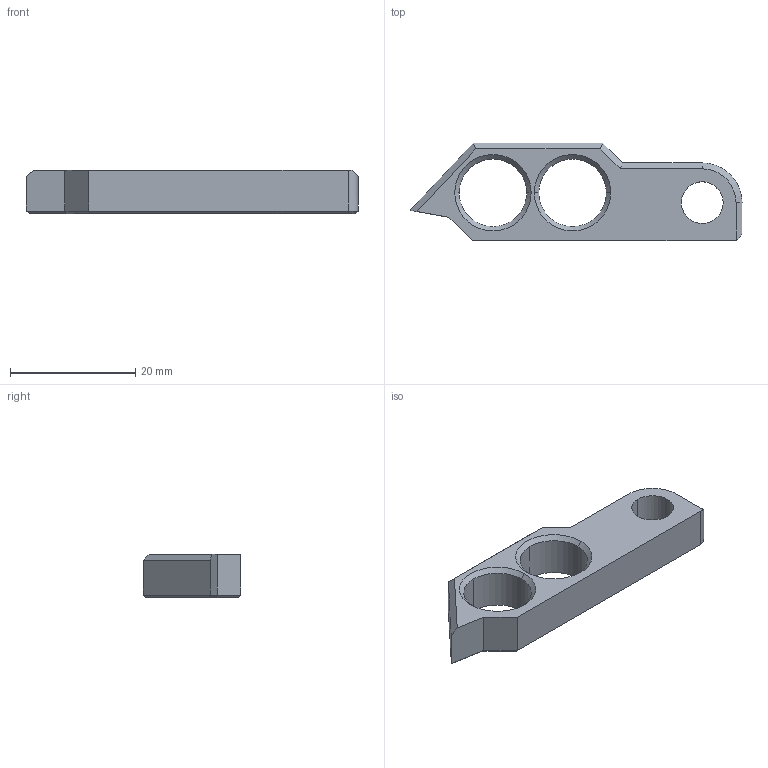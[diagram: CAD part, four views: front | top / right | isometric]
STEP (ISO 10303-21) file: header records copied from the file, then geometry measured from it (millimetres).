
FILE_DESCRIPTION (( 'STEP AP203' ), '1' );
FILE_NAME ('AF-HF-LR-PRT-005-STEP.STEP', '2020-10-04T16:10:06', ( '' ), ( '' ), 'SwSTEP 2.0', 'SolidWorks 2018', '' );
FILE_SCHEMA (( 'CONFIG_CONTROL_DESIGN' ));
Length unit declared in the file: inch
Products named in the file (1): AF-HF-LR-PRT-005-STEP
Bounding box: 52.99 x 15.62 x 6.91 mm (x, y, z)
Volume: 3028.7 mm3; surface area: 2254.9 mm2
Topology: 1 solids, 1 shells, 40 faces, 99 edges, 61 vertices
Faces by surface type: plane 23, cone 9, cylinder 8
Entity records: 1265 total; most frequent: DIRECTION 211, CARTESIAN_POINT 204, ORIENTED_EDGE 198, EDGE_CURVE 99, AXIS2_PLACEMENT_3D 72, LINE 67, VECTOR 67, VERTEX_POINT 61
